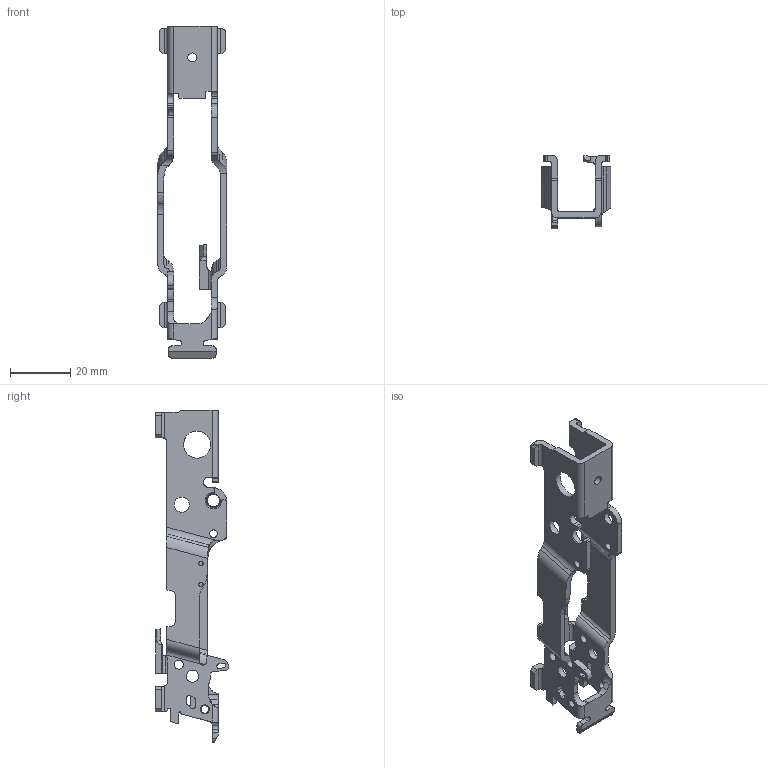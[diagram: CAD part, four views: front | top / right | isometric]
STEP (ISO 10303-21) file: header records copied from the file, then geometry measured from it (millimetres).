
FILE_DESCRIPTION(/* description */ (''),/* implementation_level */ '2;1');
FILE_NAME(/* name */ '320 FCU complete.step',/* time_stamp */ '2021-04-10T07:19:37-04:00',/* author */ (''),/* organization */ (''),/* preprocessor_version */ 'ST-DEVELOPER v18.1',/* originating_system */ 'Autodesk Translation Framework v10.6.0.1341',/* authorisation */ '');
FILE_SCHEMA (('AUTOMOTIVE_DESIGN { 1 0 10303 214 3 1 1 }'));
Length unit declared in the file: millimetre
Products named in the file (1): 320 FCU complete
Bounding box: 23.15 x 24.3 x 110.25 mm (x, y, z)
Volume: 7058.5 mm3; surface area: 8733.6 mm2
Topology: 1 solids, 1 shells, 267 faces, 792 edges, 524 vertices
Faces by surface type: plane 133, cylinder 125, cone 7, torus 2
Full cylindrical faces by diameter (mm): 1.6 x2, 2.55 x4, 3 x1, 3.03 x2, 4 x3, 5 x2, 9 x2
Entity records: 9296 total; most frequent: CARTESIAN_POINT 1847, ORIENTED_EDGE 1584, DIRECTION 1558, EDGE_CURVE 792, AXIS2_PLACEMENT_3D 530, VERTEX_POINT 524, LINE 498, VECTOR 498
